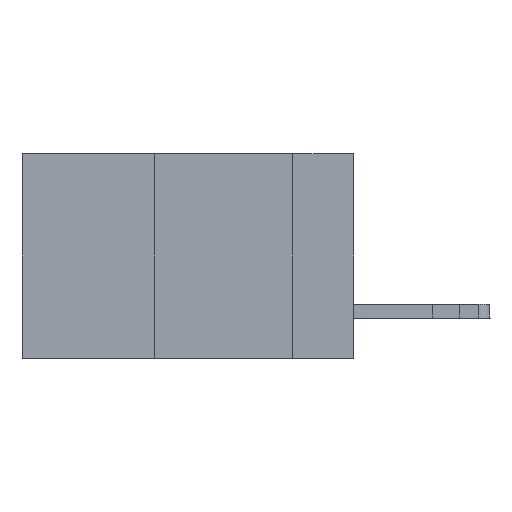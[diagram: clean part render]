
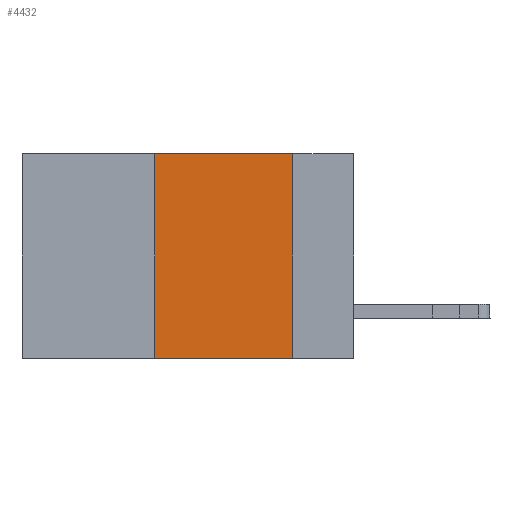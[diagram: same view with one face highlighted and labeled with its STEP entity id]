
A CAD part, left-side view. The second image highlights one B-rep face of the part: STEP entity #4432.
In plain terms, the highlighted planar face has unit normal (-1, 0, 0).
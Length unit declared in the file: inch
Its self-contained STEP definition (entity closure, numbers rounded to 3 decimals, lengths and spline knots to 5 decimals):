
#10 = CARTESIAN_POINT ( 'NONE',  ( 0., 0.36, 0. ) ) ;
#281 = VERTEX_POINT ( 'NONE', #1202 ) ;
#658 = CARTESIAN_POINT ( 'NONE',  ( 0., 0.11, -0.37 ) ) ;
#1121 = CARTESIAN_POINT ( 'NONE',  ( 0., 0.36, -0.37 ) ) ;
#1202 = CARTESIAN_POINT ( 'NONE',  ( 0., 0.11, 0. ) ) ;
#2578 = CARTESIAN_POINT ( 'NONE',  ( 0., 0.6, 0. ) ) ;
#2919 = DIRECTION ( 'NONE',  ( 1., 0., 0. ) ) ;
#3126 = VERTEX_POINT ( 'NONE', #1121 ) ;
#3442 = AXIS2_PLACEMENT_3D ( 'NONE', #2578, #2919, #6105 ) ;
#3781 = CARTESIAN_POINT ( 'NONE',  ( 0., 0.6, 0. ) ) ;
#3788 = VECTOR ( 'NONE', #9752, 39.37008 ) ;
#4432 = ADVANCED_FACE ( 'NONE', ( #14395 ), #17672, .F. ) ;
#4970 = DIRECTION ( 'NONE',  ( 0., -1., 0. ) ) ;
#5537 = DIRECTION ( 'NONE',  ( 0., -1., 0. ) ) ;
#6105 = DIRECTION ( 'NONE',  ( 0., 0., -1. ) ) ;
#6866 = EDGE_LOOP ( 'NONE', ( #7977, #19558, #19231, #20177 ) ) ;
#7091 = CARTESIAN_POINT ( 'NONE',  ( 0., 0.11, 0. ) ) ;
#7977 = ORIENTED_EDGE ( 'NONE', *, *, #16594, .F. ) ;
#8433 = VERTEX_POINT ( 'NONE', #15792 ) ;
#9752 = DIRECTION ( 'NONE',  ( 0., 0., 1. ) ) ;
#9873 = VERTEX_POINT ( 'NONE', #658 ) ;
#13918 = LINE ( 'NONE', #3781, #17450 ) ;
#14395 = FACE_OUTER_BOUND ( 'NONE', #6866, .T. ) ;
#15792 = CARTESIAN_POINT ( 'NONE',  ( 0., 0.36, 0. ) ) ;
#16594 = EDGE_CURVE ( 'NONE', #281, #9873, #20414, .T. ) ;
#16757 = VECTOR ( 'NONE', #17121, 39.37008 ) ;
#16883 = LINE ( 'NONE', #10, #3788 ) ;
#16898 = EDGE_CURVE ( 'NONE', #3126, #9873, #20166, .T. ) ;
#16939 = EDGE_CURVE ( 'NONE', #3126, #8433, #16883, .T. ) ;
#17121 = DIRECTION ( 'NONE',  ( 0., 0., -1. ) ) ;
#17450 = VECTOR ( 'NONE', #5537, 39.37008 ) ;
#17672 = PLANE ( 'NONE',  #3442 ) ;
#19231 = ORIENTED_EDGE ( 'NONE', *, *, #16939, .F. ) ;
#19558 = ORIENTED_EDGE ( 'NONE', *, *, #21430, .F. ) ;
#19739 = CARTESIAN_POINT ( 'NONE',  ( 0., 0.6, -0.37 ) ) ;
#20166 = LINE ( 'NONE', #19739, #21350 ) ;
#20177 = ORIENTED_EDGE ( 'NONE', *, *, #16898, .T. ) ;
#20414 = LINE ( 'NONE', #7091, #16757 ) ;
#21350 = VECTOR ( 'NONE', #4970, 39.37008 ) ;
#21430 = EDGE_CURVE ( 'NONE', #8433, #281, #13918, .T. ) ;
